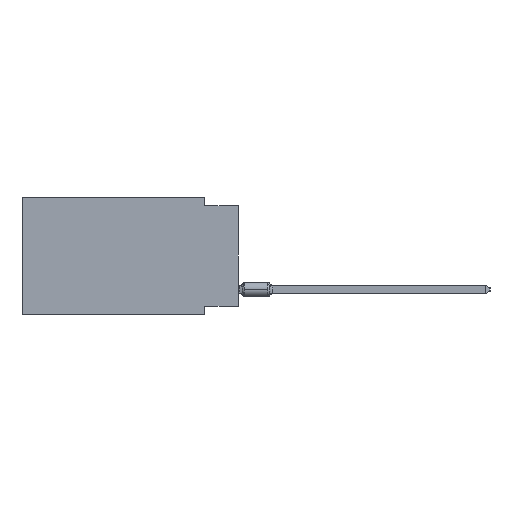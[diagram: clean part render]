
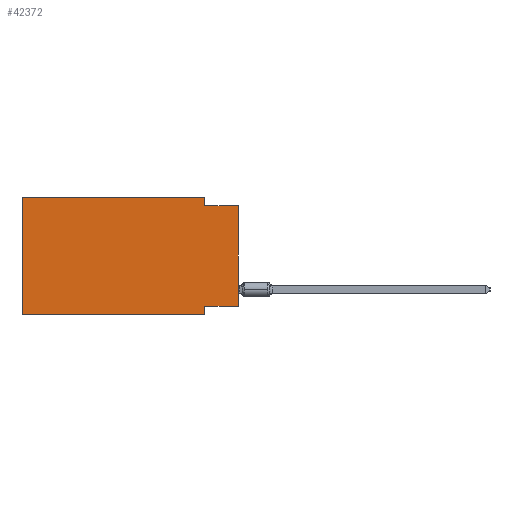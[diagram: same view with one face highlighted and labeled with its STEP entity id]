
A CAD part, left-side view. The second image highlights one B-rep face of the part: STEP entity #42372.
In plain terms, the highlighted planar face has unit normal (-1, 0, 0).
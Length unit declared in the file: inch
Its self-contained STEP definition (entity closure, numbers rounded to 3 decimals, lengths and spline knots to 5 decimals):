
#889 = EDGE_LOOP ( 'NONE', ( #25232, #25872, #12054, #20793, #7958, #20552, #33863, #27767 ) ) ;
#1067 = LINE ( 'NONE', #27009, #22795 ) ;
#1435 = CARTESIAN_POINT ( 'NONE',  ( 0., 0.1, -0.35 ) ) ;
#4258 = VERTEX_POINT ( 'NONE', #32940 ) ;
#6177 = DIRECTION ( 'NONE',  ( 1., 0., 0. ) ) ;
#6227 = DIRECTION ( 'NONE',  ( 0., 0., -1. ) ) ;
#6938 = DIRECTION ( 'NONE',  ( 0., -1., 0. ) ) ;
#7574 = CARTESIAN_POINT ( 'NONE',  ( 0., 0.645, 0. ) ) ;
#7871 = CARTESIAN_POINT ( 'NONE',  ( 0., 0., -0.025 ) ) ;
#7958 = ORIENTED_EDGE ( 'NONE', *, *, #24586, .F. ) ;
#10028 = DIRECTION ( 'NONE',  ( 0., 0., 1. ) ) ;
#12054 = ORIENTED_EDGE ( 'NONE', *, *, #46698, .F. ) ;
#12613 = EDGE_CURVE ( 'NONE', #32228, #4258, #38302, .T. ) ;
#12778 = VERTEX_POINT ( 'NONE', #24602 ) ;
#13189 = CARTESIAN_POINT ( 'NONE',  ( 0., 0.1, 0. ) ) ;
#13190 = LINE ( 'NONE', #41762, #19908 ) ;
#14842 = CARTESIAN_POINT ( 'NONE',  ( 0., 0.1, -0.025 ) ) ;
#15932 = AXIS2_PLACEMENT_3D ( 'NONE', #20810, #6177, #27536 ) ;
#16263 = CARTESIAN_POINT ( 'NONE',  ( 0., 0.645, 0. ) ) ;
#16743 = FACE_OUTER_BOUND ( 'NONE', #889, .T. ) ;
#17999 = VERTEX_POINT ( 'NONE', #13189 ) ;
#18193 = LINE ( 'NONE', #42929, #34359 ) ;
#19908 = VECTOR ( 'NONE', #6227, 39.37008 ) ;
#19927 = CARTESIAN_POINT ( 'NONE',  ( 0., 0., -0.325 ) ) ;
#20334 = PLANE ( 'NONE',  #15932 ) ;
#20552 = ORIENTED_EDGE ( 'NONE', *, *, #46961, .T. ) ;
#20793 = ORIENTED_EDGE ( 'NONE', *, *, #26895, .F. ) ;
#20810 = CARTESIAN_POINT ( 'NONE',  ( 0., 0.645, 0. ) ) ;
#21113 = CARTESIAN_POINT ( 'NONE',  ( 0., 0.645, -0.35 ) ) ;
#22736 = EDGE_CURVE ( 'NONE', #45804, #4258, #1067, .T. ) ;
#22795 = VECTOR ( 'NONE', #27735, 39.37008 ) ;
#24264 = LINE ( 'NONE', #19927, #32602 ) ;
#24586 = EDGE_CURVE ( 'NONE', #12778, #47492, #18193, .T. ) ;
#24602 = CARTESIAN_POINT ( 'NONE',  ( 0., 0.645, -0.35 ) ) ;
#25232 = ORIENTED_EDGE ( 'NONE', *, *, #22736, .T. ) ;
#25422 = EDGE_CURVE ( 'NONE', #28838, #29577, #36510, .T. ) ;
#25598 = VECTOR ( 'NONE', #30925, 39.37008 ) ;
#25872 = ORIENTED_EDGE ( 'NONE', *, *, #12613, .F. ) ;
#26895 = EDGE_CURVE ( 'NONE', #47492, #17999, #38366, .T. ) ;
#27009 = CARTESIAN_POINT ( 'NONE',  ( 0., 0., 0. ) ) ;
#27489 = DIRECTION ( 'NONE',  ( 0., -1., 0. ) ) ;
#27536 = DIRECTION ( 'NONE',  ( 0., 0., -1. ) ) ;
#27735 = DIRECTION ( 'NONE',  ( 0., 0., 1. ) ) ;
#27767 = ORIENTED_EDGE ( 'NONE', *, *, #29632, .F. ) ;
#28838 = VERTEX_POINT ( 'NONE', #43097 ) ;
#29577 = VERTEX_POINT ( 'NONE', #1435 ) ;
#29632 = EDGE_CURVE ( 'NONE', #45804, #28838, #24264, .T. ) ;
#30925 = DIRECTION ( 'NONE',  ( 0., -1., 0. ) ) ;
#32228 = VERTEX_POINT ( 'NONE', #14842 ) ;
#32602 = VECTOR ( 'NONE', #34585, 39.37008 ) ;
#32940 = CARTESIAN_POINT ( 'NONE',  ( 0., 0., -0.025 ) ) ;
#33863 = ORIENTED_EDGE ( 'NONE', *, *, #25422, .F. ) ;
#34359 = VECTOR ( 'NONE', #10028, 39.37008 ) ;
#34585 = DIRECTION ( 'NONE',  ( 0., 1., 0. ) ) ;
#36510 = LINE ( 'NONE', #40339, #45868 ) ;
#37200 = DIRECTION ( 'NONE',  ( 0., 0., -1. ) ) ;
#38302 = LINE ( 'NONE', #7871, #38722 ) ;
#38358 = VECTOR ( 'NONE', #6938, 39.37008 ) ;
#38366 = LINE ( 'NONE', #16263, #25598 ) ;
#38722 = VECTOR ( 'NONE', #27489, 39.37008 ) ;
#40339 = CARTESIAN_POINT ( 'NONE',  ( 0., 0.1, -0.35 ) ) ;
#40917 = CARTESIAN_POINT ( 'NONE',  ( 0., 0., -0.325 ) ) ;
#41762 = CARTESIAN_POINT ( 'NONE',  ( 0., 0.1, 0. ) ) ;
#42372 = ADVANCED_FACE ( 'NONE', ( #16743 ), #20334, .F. ) ;
#42929 = CARTESIAN_POINT ( 'NONE',  ( 0., 0.645, 0. ) ) ;
#43097 = CARTESIAN_POINT ( 'NONE',  ( 0., 0.1, -0.325 ) ) ;
#45804 = VERTEX_POINT ( 'NONE', #40917 ) ;
#45868 = VECTOR ( 'NONE', #37200, 39.37008 ) ;
#46698 = EDGE_CURVE ( 'NONE', #17999, #32228, #13190, .T. ) ;
#46961 = EDGE_CURVE ( 'NONE', #12778, #29577, #47033, .T. ) ;
#47033 = LINE ( 'NONE', #21113, #38358 ) ;
#47492 = VERTEX_POINT ( 'NONE', #7574 ) ;
